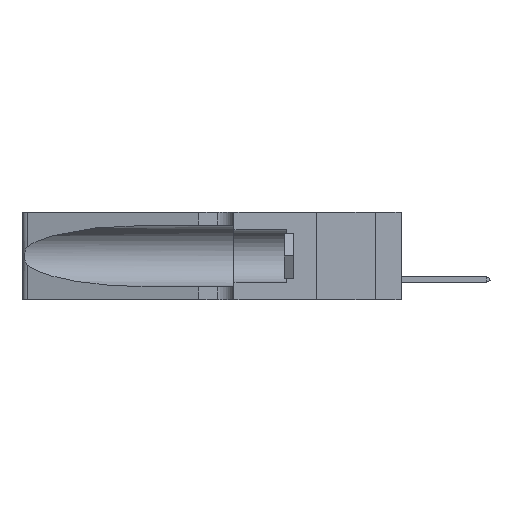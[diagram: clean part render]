
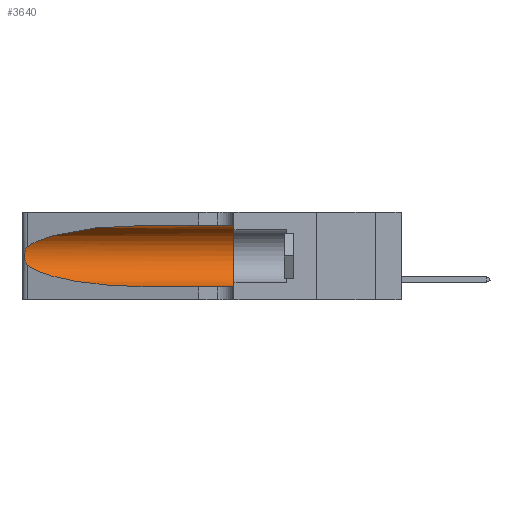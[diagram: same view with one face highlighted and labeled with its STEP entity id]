
A CAD part, left-side view. The second image highlights one B-rep face of the part: STEP entity #3640.
In plain terms, the highlighted cylindrical face has radius 3.308 mm (diameter 6.617 mm), a partial arc.
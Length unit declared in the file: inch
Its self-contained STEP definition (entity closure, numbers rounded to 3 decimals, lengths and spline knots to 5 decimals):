
#942 = LINE ( 'NONE', #42482, #35704 ) ;
#1350 = EDGE_CURVE ( 'NONE', #10866, #1612, #38703, .T. ) ;
#1612 = VERTEX_POINT ( 'NONE', #29776 ) ;
#1861 = VERTEX_POINT ( 'NONE', #34809 ) ;
#1890 = EDGE_CURVE ( 'NONE', #24399, #1861, #31719, .T. ) ;
#1997 = ORIENTED_EDGE ( 'NONE', *, *, #44789, .F. ) ;
#2255 = VERTEX_POINT ( 'NONE', #35754 ) ;
#2531 = DIRECTION ( 'NONE',  ( 0., 0., -1. ) ) ;
#2637 = CARTESIAN_POINT ( 'NONE',  ( 0.25639, 1.23184, 0.21858 ) ) ;
#2874 = CARTESIAN_POINT ( 'NONE',  ( 0.1305, 0.35, 0.05475 ) ) ;
#3640 = ADVANCED_FACE ( 'NONE', ( #18033 ), #32116, .F. ) ;
#3924 = AXIS2_PLACEMENT_3D ( 'NONE', #26965, #5415, #30723 ) ;
#5415 = DIRECTION ( 'NONE',  ( 0., 1., 0. ) ) ;
#6253 = CARTESIAN_POINT ( 'NONE',  ( 0.26017, 1.23833, 0.17102 ) ) ;
#6558 = CARTESIAN_POINT ( 'NONE',  ( 0.25787, 1.23484, 0.2124 ) ) ;
#6824 = DIRECTION ( 'NONE',  ( 0., -1., 0. ) ) ;
#8739 = EDGE_LOOP ( 'NONE', ( #29199, #26584, #20424, #20839, #1997, #19572 ) ) ;
#9161 = CARTESIAN_POINT ( 'NONE',  ( 0.1305, 1.61858, 0.31525 ) ) ;
#10146 = CARTESIAN_POINT ( 'NONE',  ( 0.25856, 1.23593, 0.16098 ) ) ;
#10866 = VERTEX_POINT ( 'NONE', #44470 ) ;
#11750 =( BOUNDED_CURVE ( )  B_SPLINE_CURVE ( 3, ( #13162, #41981, #20027, #45381 ),
 .UNSPECIFIED., .F., .T. ) 
 B_SPLINE_CURVE_WITH_KNOTS ( ( 4, 4 ),
 ( 3.44316, 4.71239 ),
 .UNSPECIFIED. ) 
 CURVE ( )  GEOMETRIC_REPRESENTATION_ITEM ( )  RATIONAL_B_SPLINE_CURVE ( ( 1., 0.87, 0.87, 1. ) ) 
 REPRESENTATION_ITEM ( '' )  );
#13162 = CARTESIAN_POINT ( 'NONE',  ( 0.25487, 1.22718, 0.14631 ) ) ;
#13612 = CARTESIAN_POINT ( 'NONE',  ( 0.1305, 1.61858, 0.185 ) ) ;
#13720 = CARTESIAN_POINT ( 'NONE',  ( 0.25639, 1.23186, 0.15144 ) ) ;
#13873 = CARTESIAN_POINT ( 'NONE',  ( 0.26075, 1.23896, 0.19203 ) ) ;
#16184 = CARTESIAN_POINT ( 'NONE',  ( 0.18966, 0.96281, 0.31525 ) ) ;
#17276 = CARTESIAN_POINT ( 'NONE',  ( 0.25555, 1.22993, 0.14849 ) ) ;
#18033 = FACE_OUTER_BOUND ( 'NONE', #8739, .T. ) ;
#19572 = ORIENTED_EDGE ( 'NONE', *, *, #1890, .F. ) ;
#20027 = CARTESIAN_POINT ( 'NONE',  ( 0.18966, 0.96281, 0.05475 ) ) ;
#20424 = ORIENTED_EDGE ( 'NONE', *, *, #26813, .T. ) ;
#20839 = ORIENTED_EDGE ( 'NONE', *, *, #45125, .T. ) ;
#23443 = CARTESIAN_POINT ( 'NONE',  ( 0.25487, 1.22718, 0.22369 ) ) ;
#23699 = DIRECTION ( 'NONE',  ( 0., -1., 0. ) ) ;
#24399 = VERTEX_POINT ( 'NONE', #39240 ) ;
#24678 = CARTESIAN_POINT ( 'NONE',  ( 0.26018, 1.23835, 0.19895 ) ) ;
#26584 = ORIENTED_EDGE ( 'NONE', *, *, #1350, .T. ) ;
#26813 = EDGE_CURVE ( 'NONE', #1612, #2255, #11750, .T. ) ;
#26965 = CARTESIAN_POINT ( 'NONE',  ( 0.1305, 0.35, 0.185 ) ) ;
#27612 = CARTESIAN_POINT ( 'NONE',  ( 0.25854, 1.2359, 0.20912 ) ) ;
#27987 = DIRECTION ( 'NONE',  ( 0., -1., 0. ) ) ;
#29199 = ORIENTED_EDGE ( 'NONE', *, *, #38802, .T. ) ;
#29776 = CARTESIAN_POINT ( 'NONE',  ( 0.25487, 1.22718, 0.14631 ) ) ;
#30723 = DIRECTION ( 'NONE',  ( 0., 0., 1. ) ) ;
#31563 = CARTESIAN_POINT ( 'NONE',  ( 0.26075, 1.23896, 0.178 ) ) ;
#31719 = LINE ( 'NONE', #9161, #42927 ) ;
#32116 = CYLINDRICAL_SURFACE ( 'NONE', #33885, 0.13025 ) ;
#33885 = AXIS2_PLACEMENT_3D ( 'NONE', #13612, #27987, #2531 ) ;
#34809 = CARTESIAN_POINT ( 'NONE',  ( 0.1305, 0.35, 0.31525 ) ) ;
#34876 = CARTESIAN_POINT ( 'NONE',  ( 0.25789, 1.23486, 0.15765 ) ) ;
#35328 =( BOUNDED_CURVE ( )  B_SPLINE_CURVE ( 3, ( #37695, #16184, #44847, #23443 ),
 .UNSPECIFIED., .F., .T. ) 
 B_SPLINE_CURVE_WITH_KNOTS ( ( 4, 4 ),
 ( 1.5708, 2.84003 ),
 .UNSPECIFIED. ) 
 CURVE ( )  GEOMETRIC_REPRESENTATION_ITEM ( )  RATIONAL_B_SPLINE_CURVE ( ( 1., 0.87, 0.87, 1. ) ) 
 REPRESENTATION_ITEM ( '' )  );
#35351 = CARTESIAN_POINT ( 'NONE',  ( 0.25487, 1.22718, 0.22369 ) ) ;
#35704 = VECTOR ( 'NONE', #6824, 39.37008 ) ;
#35754 = CARTESIAN_POINT ( 'NONE',  ( 0.1305, 0.72297, 0.05475 ) ) ;
#37695 = CARTESIAN_POINT ( 'NONE',  ( 0.1305, 0.72297, 0.31525 ) ) ;
#38703 = B_SPLINE_CURVE_WITH_KNOTS ( 'NONE', 3,
 ( #35351, #45477, #2637, #6558, #27612, #24678, #13873, #31563, #6253, #10146, #34876, #13720, #17276, #38942 ),
 .UNSPECIFIED., .F., .F.,
 ( 4, 2, 2, 2, 2, 2, 4 ),
 ( 0., 0.00027, 0.00053, 0.00107, 0.0016, 0.00187, 0.00214 ),
 .UNSPECIFIED. ) ;
#38802 = EDGE_CURVE ( 'NONE', #24399, #10866, #35328, .T. ) ;
#38942 = CARTESIAN_POINT ( 'NONE',  ( 0.25487, 1.22718, 0.14631 ) ) ;
#39240 = CARTESIAN_POINT ( 'NONE',  ( 0.1305, 0.72297, 0.31525 ) ) ;
#41981 = CARTESIAN_POINT ( 'NONE',  ( 0.2373, 1.15595, 0.08982 ) ) ;
#42482 = CARTESIAN_POINT ( 'NONE',  ( 0.1305, 1.61858, 0.05475 ) ) ;
#42927 = VECTOR ( 'NONE', #23699, 39.37008 ) ;
#44470 = CARTESIAN_POINT ( 'NONE',  ( 0.25487, 1.22718, 0.22369 ) ) ;
#44789 = EDGE_CURVE ( 'NONE', #1861, #45446, #45201, .T. ) ;
#44847 = CARTESIAN_POINT ( 'NONE',  ( 0.2373, 1.15595, 0.28018 ) ) ;
#45125 = EDGE_CURVE ( 'NONE', #2255, #45446, #942, .T. ) ;
#45201 = CIRCLE ( 'NONE', #3924, 0.13025 ) ;
#45381 = CARTESIAN_POINT ( 'NONE',  ( 0.1305, 0.72297, 0.05475 ) ) ;
#45446 = VERTEX_POINT ( 'NONE', #2874 ) ;
#45477 = CARTESIAN_POINT ( 'NONE',  ( 0.25555, 1.22994, 0.2215 ) ) ;
